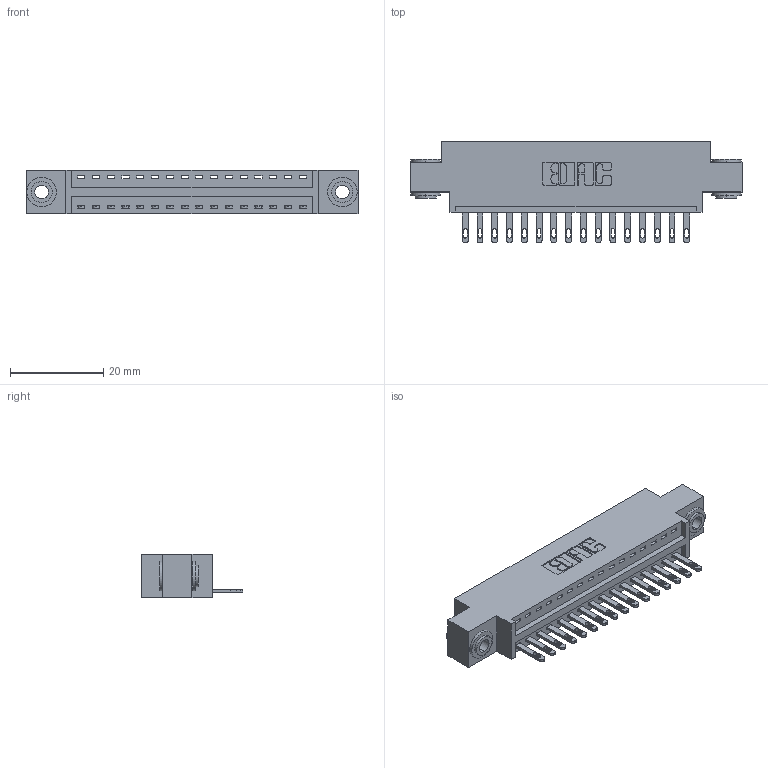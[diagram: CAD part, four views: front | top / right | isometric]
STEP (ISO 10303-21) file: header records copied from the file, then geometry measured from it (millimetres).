
FILE_DESCRIPTION (( 'STEP AP203' ), '1' );
FILE_NAME ('896-016-500-603.STEP', '2021-07-27T15:42:24', ( '' ), ( '' ), 'SwSTEP 2.0', 'SolidWorks 2020', '' );
FILE_SCHEMA (( 'CONFIG_CONTROL_DESIGN' ));
Length unit declared in the file: inch
Products named in the file (4): 345-292-001_345-293-100; 345-250-002_345-250-002-102; 896-016-500-603; 846 Part_0.170 Offset - 0.156 Dia-TH
Assembly tree (19 placements, depth 2):
  896-016-500-603
    846 Part_0.170 Offset - 0.156 Dia-TH
    345-292-001_345-293-100  x16
    345-250-002_345-250-002-102  x2
Bounding box: 71.37 x 21.84 x 9.4 mm (x, y, z)
Volume: 6527.6 mm3; surface area: 8294.9 mm2
Topology: 19 solids, 19 shells, 1028 faces, 3105 edges, 2066 vertices
Faces by surface type: plane 634, cylinder 386, cone 8
Entity records: 14142 total; most frequent: CARTESIAN_POINT 2411, ORIENTED_EDGE 2354, DIRECTION 2191, EDGE_CURVE 1177, VECTOR 953, LINE 953, VERTEX_POINT 782, AXIS2_PLACEMENT_3D 619
